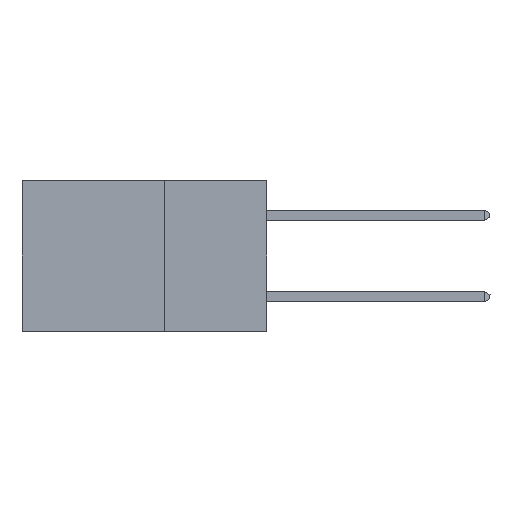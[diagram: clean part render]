
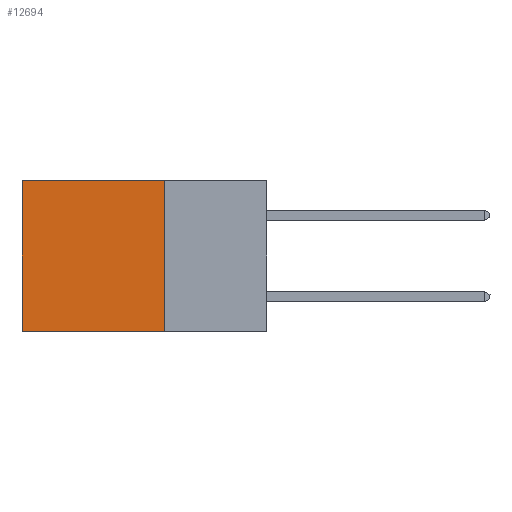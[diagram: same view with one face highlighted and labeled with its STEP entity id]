
A CAD part, left-side view. The second image highlights one B-rep face of the part: STEP entity #12694.
In plain terms, the highlighted planar face has unit normal (-1, 0, 0).
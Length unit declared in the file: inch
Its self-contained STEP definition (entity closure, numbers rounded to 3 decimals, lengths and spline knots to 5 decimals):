
#132 = CARTESIAN_POINT ( 'NONE',  ( 0.2875, 0.25, -0.37 ) ) ;
#278 = PLANE ( 'NONE',  #5091 ) ;
#342 = DIRECTION ( 'NONE',  ( 1., 0., 0. ) ) ;
#792 = DIRECTION ( 'NONE',  ( 0., 1., 0. ) ) ;
#1346 = FACE_OUTER_BOUND ( 'NONE', #5946, .T. ) ;
#1594 = CARTESIAN_POINT ( 'NONE',  ( 0.2875, 0.6, -0.37 ) ) ;
#2158 = DIRECTION ( 'NONE',  ( 0., 1., 0. ) ) ;
#2408 = DIRECTION ( 'NONE',  ( 0., 0., -1. ) ) ;
#2729 = CARTESIAN_POINT ( 'NONE',  ( 0.2875, 0.25, -0.37 ) ) ;
#2799 = VERTEX_POINT ( 'NONE', #1594 ) ;
#3265 = CARTESIAN_POINT ( 'NONE',  ( 0.2875, 0.25, 0. ) ) ;
#3301 = ORIENTED_EDGE ( 'NONE', *, *, #10305, .T. ) ;
#3459 = ORIENTED_EDGE ( 'NONE', *, *, #3973, .F. ) ;
#3973 = EDGE_CURVE ( 'NONE', #6025, #2799, #12297, .T. ) ;
#3992 = CARTESIAN_POINT ( 'NONE',  ( 0.2875, 0.25, 0. ) ) ;
#4067 = VERTEX_POINT ( 'NONE', #4213 ) ;
#4213 = CARTESIAN_POINT ( 'NONE',  ( 0.2875, 0.6, 0. ) ) ;
#4717 = VECTOR ( 'NONE', #2408, 39.37008 ) ;
#5091 = AXIS2_PLACEMENT_3D ( 'NONE', #6648, #342, #5582 ) ;
#5582 = DIRECTION ( 'NONE',  ( 0., 0., -1. ) ) ;
#5946 = EDGE_LOOP ( 'NONE', ( #6131, #3459, #9692, #3301 ) ) ;
#6025 = VERTEX_POINT ( 'NONE', #2729 ) ;
#6131 = ORIENTED_EDGE ( 'NONE', *, *, #11386, .T. ) ;
#6546 = VECTOR ( 'NONE', #8401, 39.37008 ) ;
#6648 = CARTESIAN_POINT ( 'NONE',  ( 0.2875, 0.25, 0. ) ) ;
#8401 = DIRECTION ( 'NONE',  ( 0., 0., -1. ) ) ;
#8454 = CARTESIAN_POINT ( 'NONE',  ( 0.2875, 0.25, 0. ) ) ;
#8803 = EDGE_CURVE ( 'NONE', #9268, #6025, #9460, .T. ) ;
#8852 = VECTOR ( 'NONE', #2158, 39.37008 ) ;
#9268 = VERTEX_POINT ( 'NONE', #3265 ) ;
#9460 = LINE ( 'NONE', #8454, #4717 ) ;
#9692 = ORIENTED_EDGE ( 'NONE', *, *, #8803, .F. ) ;
#10305 = EDGE_CURVE ( 'NONE', #9268, #4067, #13196, .T. ) ;
#10632 = VECTOR ( 'NONE', #792, 39.37008 ) ;
#11386 = EDGE_CURVE ( 'NONE', #4067, #2799, #12490, .T. ) ;
#12297 = LINE ( 'NONE', #132, #8852 ) ;
#12490 = LINE ( 'NONE', #12809, #6546 ) ;
#12694 = ADVANCED_FACE ( 'NONE', ( #1346 ), #278, .F. ) ;
#12809 = CARTESIAN_POINT ( 'NONE',  ( 0.2875, 0.6, 0. ) ) ;
#13196 = LINE ( 'NONE', #3992, #10632 ) ;
